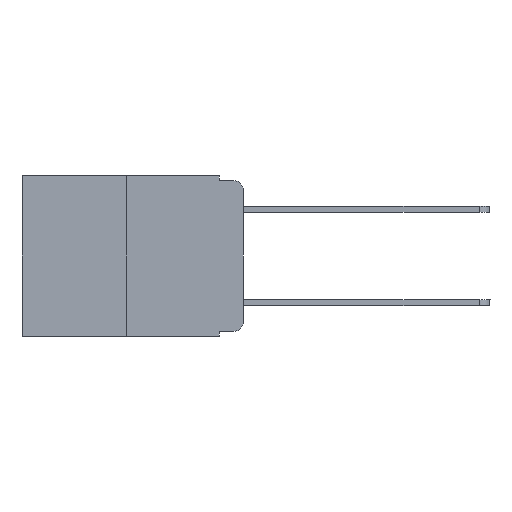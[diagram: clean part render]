
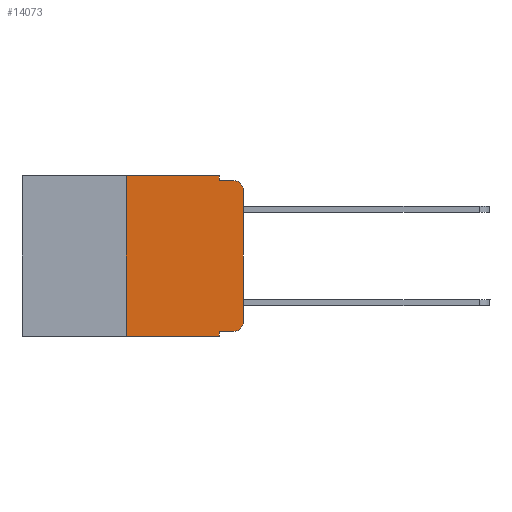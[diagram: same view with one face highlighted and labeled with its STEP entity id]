
A CAD part, left-side view. The second image highlights one B-rep face of the part: STEP entity #14073.
In plain terms, the highlighted planar face has unit normal (-1, 0, 0).
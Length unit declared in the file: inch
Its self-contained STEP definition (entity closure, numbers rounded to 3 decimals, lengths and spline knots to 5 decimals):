
#339 = CARTESIAN_POINT ( 'NONE',  ( 0., 0.25, 0. ) ) ;
#519 = DIRECTION ( 'NONE',  ( -1., 0., 0. ) ) ;
#1178 = DIRECTION ( 'NONE',  ( 0., 0., 1. ) ) ;
#1252 = DIRECTION ( 'NONE',  ( 0., -1., 0. ) ) ;
#1400 = EDGE_CURVE ( 'NONE', #18919, #11998, #12562, .T. ) ;
#1487 = CARTESIAN_POINT ( 'NONE',  ( 0., 0.051, -0.333 ) ) ;
#1534 = ORIENTED_EDGE ( 'NONE', *, *, #5270, .T. ) ;
#1858 = VECTOR ( 'NONE', #13891, 39.37008 ) ;
#2197 = VERTEX_POINT ( 'NONE', #16790 ) ;
#2539 = VERTEX_POINT ( 'NONE', #11517 ) ;
#3162 = DIRECTION ( 'NONE',  ( 0., 0., -1. ) ) ;
#3318 = DIRECTION ( 'NONE',  ( 1., 0., 0. ) ) ;
#3640 = CARTESIAN_POINT ( 'NONE',  ( 0., 0.051, -0.343 ) ) ;
#3728 = DIRECTION ( 'NONE',  ( 0., 0., -1. ) ) ;
#3874 = ORIENTED_EDGE ( 'NONE', *, *, #13029, .F. ) ;
#3948 = VECTOR ( 'NONE', #12266, 39.37008 ) ;
#5145 = DIRECTION ( 'NONE',  ( 0., -1., 0. ) ) ;
#5270 = EDGE_CURVE ( 'NONE', #2197, #16591, #19698, .T. ) ;
#5371 = CARTESIAN_POINT ( 'NONE',  ( 0., 0., -0.313 ) ) ;
#5409 = AXIS2_PLACEMENT_3D ( 'NONE', #16329, #5655, #14644 ) ;
#5655 = DIRECTION ( 'NONE',  ( -1., 0., 0. ) ) ;
#5672 = VERTEX_POINT ( 'NONE', #17254 ) ;
#5702 = EDGE_CURVE ( 'NONE', #18919, #14853, #8383, .T. ) ;
#5979 = DIRECTION ( 'NONE',  ( 0., -1., 0. ) ) ;
#6052 = EDGE_CURVE ( 'NONE', #15146, #2197, #15153, .T. ) ;
#6602 = CARTESIAN_POINT ( 'NONE',  ( 0., 0.473, 0. ) ) ;
#6879 = ORIENTED_EDGE ( 'NONE', *, *, #1400, .F. ) ;
#7353 = ORIENTED_EDGE ( 'NONE', *, *, #14066, .F. ) ;
#7377 = CARTESIAN_POINT ( 'NONE',  ( 0., 0.051, -0.01 ) ) ;
#7713 = VECTOR ( 'NONE', #5979, 39.37008 ) ;
#8115 = VECTOR ( 'NONE', #5145, 39.37008 ) ;
#8383 = LINE ( 'NONE', #14176, #14032 ) ;
#8958 = ORIENTED_EDGE ( 'NONE', *, *, #11928, .F. ) ;
#9005 = CARTESIAN_POINT ( 'NONE',  ( 0., 0.051, -0.333 ) ) ;
#9257 = VERTEX_POINT ( 'NONE', #17976 ) ;
#9924 = ORIENTED_EDGE ( 'NONE', *, *, #6052, .T. ) ;
#9952 = VECTOR ( 'NONE', #1178, 39.37008 ) ;
#10352 = LINE ( 'NONE', #16601, #19032 ) ;
#11139 = CARTESIAN_POINT ( 'NONE',  ( 0., 0.25, -0.343 ) ) ;
#11413 = EDGE_CURVE ( 'NONE', #16591, #2539, #15151, .T. ) ;
#11517 = CARTESIAN_POINT ( 'NONE',  ( 0., 0., -0.03 ) ) ;
#11928 = EDGE_CURVE ( 'NONE', #11998, #9257, #10352, .T. ) ;
#11998 = VERTEX_POINT ( 'NONE', #339 ) ;
#12233 = CARTESIAN_POINT ( 'NONE',  ( 0., 0.051, 0. ) ) ;
#12266 = DIRECTION ( 'NONE',  ( 0., 0., 1. ) ) ;
#12343 = ORIENTED_EDGE ( 'NONE', *, *, #17765, .F. ) ;
#12562 = LINE ( 'NONE', #17143, #3948 ) ;
#12923 = ORIENTED_EDGE ( 'NONE', *, *, #15886, .T. ) ;
#13029 = EDGE_CURVE ( 'NONE', #15146, #14853, #13838, .T. ) ;
#13657 = CARTESIAN_POINT ( 'NONE',  ( 0., 0., 0. ) ) ;
#13838 = LINE ( 'NONE', #12233, #17472 ) ;
#13891 = DIRECTION ( 'NONE',  ( 0., 0., -1. ) ) ;
#14032 = VECTOR ( 'NONE', #17544, 39.37008 ) ;
#14066 = EDGE_CURVE ( 'NONE', #9257, #19312, #15481, .T. ) ;
#14073 = ADVANCED_FACE ( 'NONE', ( #14074 ), #15786, .F. ) ;
#14074 = FACE_OUTER_BOUND ( 'NONE', #14252, .T. ) ;
#14176 = CARTESIAN_POINT ( 'NONE',  ( 0., 0.473, -0.343 ) ) ;
#14182 = CARTESIAN_POINT ( 'NONE',  ( 0., 0.051, 0. ) ) ;
#14252 = EDGE_LOOP ( 'NONE', ( #17834, #12923, #12343, #7353, #8958, #6879, #16628, #3874, #9924, #1534 ) ) ;
#14644 = DIRECTION ( 'NONE',  ( 0., 0., -1. ) ) ;
#14853 = VERTEX_POINT ( 'NONE', #3640 ) ;
#14937 = AXIS2_PLACEMENT_3D ( 'NONE', #15894, #519, #3728 ) ;
#15146 = VERTEX_POINT ( 'NONE', #9005 ) ;
#15151 = LINE ( 'NONE', #13657, #9952 ) ;
#15153 = LINE ( 'NONE', #1487, #8115 ) ;
#15481 = LINE ( 'NONE', #14182, #1858 ) ;
#15613 = CIRCLE ( 'NONE', #5409, 0.02 ) ;
#15786 = PLANE ( 'NONE',  #19664 ) ;
#15886 = EDGE_CURVE ( 'NONE', #2539, #5672, #15613, .T. ) ;
#15894 = CARTESIAN_POINT ( 'NONE',  ( 0., 0.02, -0.313 ) ) ;
#16329 = CARTESIAN_POINT ( 'NONE',  ( 0., 0.02, -0.03 ) ) ;
#16591 = VERTEX_POINT ( 'NONE', #5371 ) ;
#16601 = CARTESIAN_POINT ( 'NONE',  ( 0., 0.473, 0. ) ) ;
#16628 = ORIENTED_EDGE ( 'NONE', *, *, #5702, .T. ) ;
#16790 = CARTESIAN_POINT ( 'NONE',  ( 0., 0.02, -0.333 ) ) ;
#17066 = DIRECTION ( 'NONE',  ( 0., 0., -1. ) ) ;
#17143 = CARTESIAN_POINT ( 'NONE',  ( 0., 0.25, 0. ) ) ;
#17254 = CARTESIAN_POINT ( 'NONE',  ( 0., 0.02, -0.01 ) ) ;
#17472 = VECTOR ( 'NONE', #3162, 39.37008 ) ;
#17544 = DIRECTION ( 'NONE',  ( 0., -1., 0. ) ) ;
#17765 = EDGE_CURVE ( 'NONE', #19312, #5672, #19547, .T. ) ;
#17834 = ORIENTED_EDGE ( 'NONE', *, *, #11413, .T. ) ;
#17976 = CARTESIAN_POINT ( 'NONE',  ( 0., 0.051, 0. ) ) ;
#18841 = CARTESIAN_POINT ( 'NONE',  ( 0., 0.051, -0.01 ) ) ;
#18919 = VERTEX_POINT ( 'NONE', #11139 ) ;
#19032 = VECTOR ( 'NONE', #1252, 39.37008 ) ;
#19312 = VERTEX_POINT ( 'NONE', #18841 ) ;
#19547 = LINE ( 'NONE', #7377, #7713 ) ;
#19664 = AXIS2_PLACEMENT_3D ( 'NONE', #6602, #3318, #17066 ) ;
#19698 = CIRCLE ( 'NONE', #14937, 0.02 ) ;
